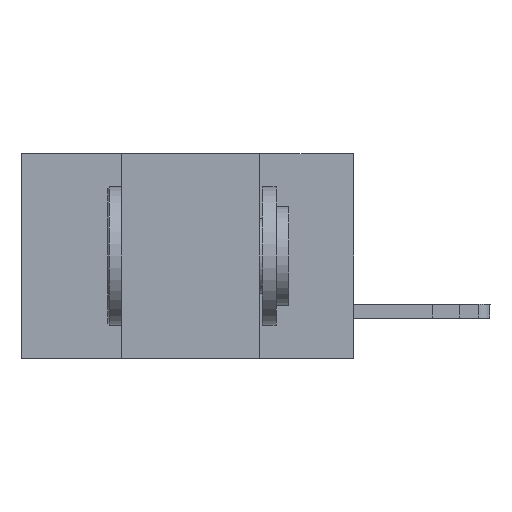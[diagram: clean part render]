
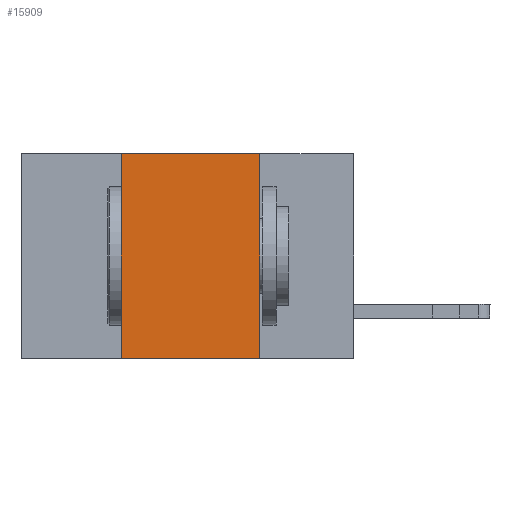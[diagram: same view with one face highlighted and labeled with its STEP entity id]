
A CAD part, left-side view. The second image highlights one B-rep face of the part: STEP entity #15909.
In plain terms, the highlighted planar face has unit normal (-1, 0, 0).
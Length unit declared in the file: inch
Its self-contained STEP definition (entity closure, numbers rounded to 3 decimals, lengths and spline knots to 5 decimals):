
#237 = CARTESIAN_POINT ( 'NONE',  ( 0., 0.6, -0.37 ) ) ;
#474 = VECTOR ( 'NONE', #9996, 39.37008 ) ;
#587 = VECTOR ( 'NONE', #18452, 39.37008 ) ;
#1151 = VECTOR ( 'NONE', #26747, 39.37008 ) ;
#2404 = EDGE_LOOP ( 'NONE', ( #20306, #18485, #14434, #20381 ) ) ;
#3185 = CARTESIAN_POINT ( 'NONE',  ( 0., 0.42, 0. ) ) ;
#3817 = CARTESIAN_POINT ( 'NONE',  ( 0., 0.6, 0. ) ) ;
#5269 = FACE_OUTER_BOUND ( 'NONE', #2404, .T. ) ;
#5535 = EDGE_CURVE ( 'NONE', #28717, #12921, #23084, .T. ) ;
#6178 = LINE ( 'NONE', #3817, #1151 ) ;
#6960 = EDGE_CURVE ( 'NONE', #22919, #28626, #17158, .T. ) ;
#9996 = DIRECTION ( 'NONE',  ( 0., -1., 0. ) ) ;
#11297 = EDGE_CURVE ( 'NONE', #28626, #28717, #6178, .T. ) ;
#11309 = AXIS2_PLACEMENT_3D ( 'NONE', #12354, #24281, #17500 ) ;
#11998 = VECTOR ( 'NONE', #19174, 39.37008 ) ;
#12354 = CARTESIAN_POINT ( 'NONE',  ( 0., 0.6, 0. ) ) ;
#12921 = VERTEX_POINT ( 'NONE', #24771 ) ;
#14434 = ORIENTED_EDGE ( 'NONE', *, *, #6960, .F. ) ;
#14443 = LINE ( 'NONE', #237, #474 ) ;
#14942 = PLANE ( 'NONE',  #11309 ) ;
#15909 = ADVANCED_FACE ( 'NONE', ( #5269 ), #14942, .F. ) ;
#16028 = CARTESIAN_POINT ( 'NONE',  ( 0., 0.42, 0. ) ) ;
#17158 = LINE ( 'NONE', #3185, #11998 ) ;
#17500 = DIRECTION ( 'NONE',  ( 0., 0., -1. ) ) ;
#18296 = CARTESIAN_POINT ( 'NONE',  ( 0., 0.42, -0.37 ) ) ;
#18452 = DIRECTION ( 'NONE',  ( 0., 0., -1. ) ) ;
#18485 = ORIENTED_EDGE ( 'NONE', *, *, #11297, .F. ) ;
#19174 = DIRECTION ( 'NONE',  ( 0., 0., 1. ) ) ;
#20306 = ORIENTED_EDGE ( 'NONE', *, *, #5535, .F. ) ;
#20381 = ORIENTED_EDGE ( 'NONE', *, *, #25256, .T. ) ;
#22919 = VERTEX_POINT ( 'NONE', #18296 ) ;
#23084 = LINE ( 'NONE', #27995, #587 ) ;
#24281 = DIRECTION ( 'NONE',  ( 1., 0., 0. ) ) ;
#24771 = CARTESIAN_POINT ( 'NONE',  ( 0., 0.17, -0.37 ) ) ;
#25256 = EDGE_CURVE ( 'NONE', #22919, #12921, #14443, .T. ) ;
#26164 = CARTESIAN_POINT ( 'NONE',  ( 0., 0.17, 0. ) ) ;
#26747 = DIRECTION ( 'NONE',  ( 0., -1., 0. ) ) ;
#27995 = CARTESIAN_POINT ( 'NONE',  ( 0., 0.17, 0. ) ) ;
#28626 = VERTEX_POINT ( 'NONE', #16028 ) ;
#28717 = VERTEX_POINT ( 'NONE', #26164 ) ;
